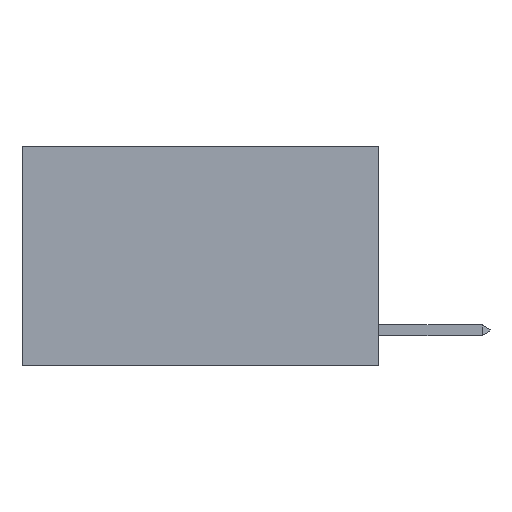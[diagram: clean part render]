
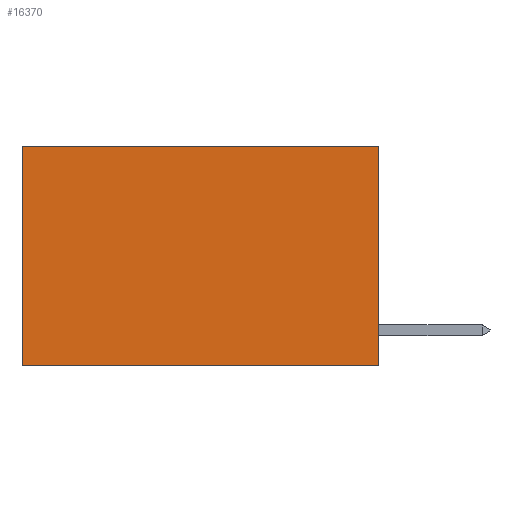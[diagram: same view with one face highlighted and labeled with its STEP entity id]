
A CAD part, left-side view. The second image highlights one B-rep face of the part: STEP entity #16370.
In plain terms, the highlighted planar face has unit normal (-1, 0, 0).
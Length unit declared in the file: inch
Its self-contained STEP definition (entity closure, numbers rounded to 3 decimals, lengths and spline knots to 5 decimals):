
#279 = CARTESIAN_POINT ( 'NONE',  ( 0.2625, 0., -0.37 ) ) ;
#2364 = EDGE_CURVE ( 'NONE', #11341, #15357, #11405, .T. ) ;
#2389 = CARTESIAN_POINT ( 'NONE',  ( 0.2625, 0., 0. ) ) ;
#3120 = VECTOR ( 'NONE', #18593, 39.37008 ) ;
#3908 = ORIENTED_EDGE ( 'NONE', *, *, #20702, .T. ) ;
#4241 = VECTOR ( 'NONE', #13430, 39.37008 ) ;
#6946 = VERTEX_POINT ( 'NONE', #15900 ) ;
#7205 = LINE ( 'NONE', #22589, #23171 ) ;
#8233 = DIRECTION ( 'NONE',  ( 0., 1., 0. ) ) ;
#9034 = DIRECTION ( 'NONE',  ( 0., 0., -1. ) ) ;
#10569 = ORIENTED_EDGE ( 'NONE', *, *, #16035, .F. ) ;
#11115 = PLANE ( 'NONE',  #16503 ) ;
#11341 = VERTEX_POINT ( 'NONE', #14714 ) ;
#11405 = LINE ( 'NONE', #279, #4241 ) ;
#11775 = DIRECTION ( 'NONE',  ( 0., 0., -1. ) ) ;
#11956 = LINE ( 'NONE', #16799, #16992 ) ;
#13430 = DIRECTION ( 'NONE',  ( 0., 1., 0. ) ) ;
#14714 = CARTESIAN_POINT ( 'NONE',  ( 0.2625, 0., -0.37 ) ) ;
#15357 = VERTEX_POINT ( 'NONE', #25419 ) ;
#15830 = EDGE_LOOP ( 'NONE', ( #23143, #23766, #10569, #3908 ) ) ;
#15900 = CARTESIAN_POINT ( 'NONE',  ( 0.2625, 0.6, 0. ) ) ;
#16035 = EDGE_CURVE ( 'NONE', #18358, #11341, #20461, .T. ) ;
#16370 = ADVANCED_FACE ( 'NONE', ( #27641 ), #11115, .F. ) ;
#16405 = CARTESIAN_POINT ( 'NONE',  ( 0.2625, 0., 0. ) ) ;
#16503 = AXIS2_PLACEMENT_3D ( 'NONE', #2389, #22029, #9034 ) ;
#16799 = CARTESIAN_POINT ( 'NONE',  ( 0.2625, 0., 0. ) ) ;
#16992 = VECTOR ( 'NONE', #8233, 39.37008 ) ;
#18358 = VERTEX_POINT ( 'NONE', #26992 ) ;
#18593 = DIRECTION ( 'NONE',  ( 0., 0., -1. ) ) ;
#20461 = LINE ( 'NONE', #16405, #3120 ) ;
#20702 = EDGE_CURVE ( 'NONE', #18358, #6946, #11956, .T. ) ;
#22029 = DIRECTION ( 'NONE',  ( 1., 0., 0. ) ) ;
#22589 = CARTESIAN_POINT ( 'NONE',  ( 0.2625, 0.6, 0. ) ) ;
#23143 = ORIENTED_EDGE ( 'NONE', *, *, #25215, .T. ) ;
#23171 = VECTOR ( 'NONE', #11775, 39.37008 ) ;
#23766 = ORIENTED_EDGE ( 'NONE', *, *, #2364, .F. ) ;
#25215 = EDGE_CURVE ( 'NONE', #6946, #15357, #7205, .T. ) ;
#25419 = CARTESIAN_POINT ( 'NONE',  ( 0.2625, 0.6, -0.37 ) ) ;
#26992 = CARTESIAN_POINT ( 'NONE',  ( 0.2625, 0., 0. ) ) ;
#27641 = FACE_OUTER_BOUND ( 'NONE', #15830, .T. ) ;
